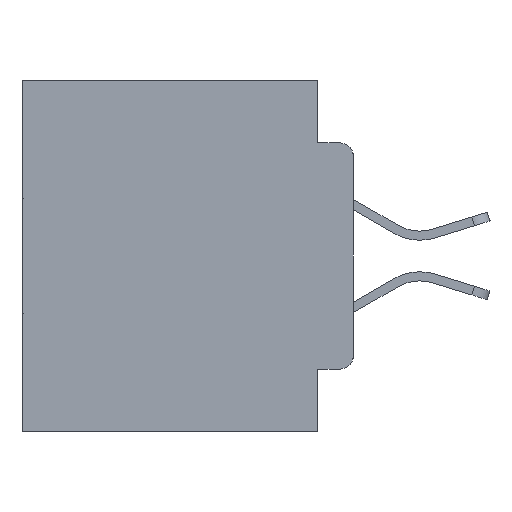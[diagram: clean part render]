
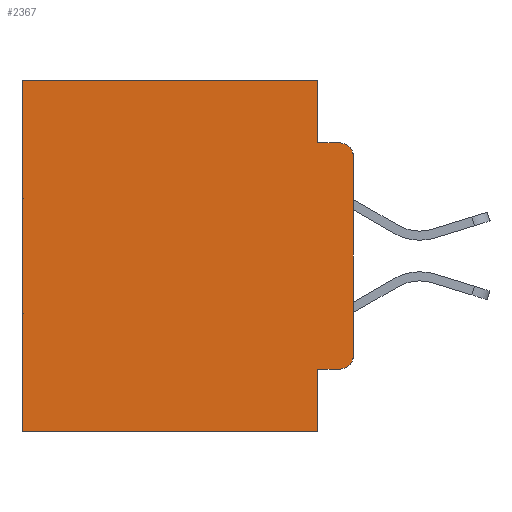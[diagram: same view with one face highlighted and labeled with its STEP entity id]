
A CAD part, left-side view. The second image highlights one B-rep face of the part: STEP entity #2367.
In plain terms, the highlighted planar face has unit normal (-1, 0, 0).
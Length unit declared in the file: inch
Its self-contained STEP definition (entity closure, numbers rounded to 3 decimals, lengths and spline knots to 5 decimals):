
#1033 = VECTOR ( 'NONE', #5697, 39.37008 ) ;
#1277 = EDGE_CURVE ( 'NONE', #19960, #2968, #4929, .T. ) ;
#1379 = CARTESIAN_POINT ( 'NONE',  ( 0.298, 0.051, 0. ) ) ;
#1910 = LINE ( 'NONE', #29981, #6306 ) ;
#2284 = ORIENTED_EDGE ( 'NONE', *, *, #23521, .T. ) ;
#2367 = ADVANCED_FACE ( 'NONE', ( #18465 ), #13854, .F. ) ;
#2561 = EDGE_CURVE ( 'NONE', #17976, #5956, #28846, .T. ) ;
#2610 = DIRECTION ( 'NONE',  ( -1., 0., 0. ) ) ;
#2968 = VERTEX_POINT ( 'NONE', #10141 ) ;
#3002 = AXIS2_PLACEMENT_3D ( 'NONE', #29935, #8965, #18314 ) ;
#3063 = VERTEX_POINT ( 'NONE', #20536 ) ;
#4716 = DIRECTION ( 'NONE',  ( -1., 0., 0. ) ) ;
#4929 = CIRCLE ( 'NONE', #16706, 0.02 ) ;
#5697 = DIRECTION ( 'NONE',  ( 0., 0., -1. ) ) ;
#5956 = VERTEX_POINT ( 'NONE', #21633 ) ;
#6157 = LINE ( 'NONE', #19961, #22907 ) ;
#6292 = EDGE_LOOP ( 'NONE', ( #26105, #29498, #7298, #27615, #23165, #8269, #11264, #27363, #2284, #11113 ) ) ;
#6306 = VECTOR ( 'NONE', #11306, 39.37008 ) ;
#6363 = CARTESIAN_POINT ( 'NONE',  ( 0.298, 0.051, -0.0885 ) ) ;
#6439 = CARTESIAN_POINT ( 'NONE',  ( 0.298, 0.051, 0. ) ) ;
#7035 = DIRECTION ( 'NONE',  ( 0., 0., -1. ) ) ;
#7298 = ORIENTED_EDGE ( 'NONE', *, *, #22353, .F. ) ;
#7480 = VERTEX_POINT ( 'NONE', #16252 ) ;
#8063 = VECTOR ( 'NONE', #23397, 39.37008 ) ;
#8269 = ORIENTED_EDGE ( 'NONE', *, *, #20281, .T. ) ;
#8716 = CARTESIAN_POINT ( 'NONE',  ( 0.298, 0., 0. ) ) ;
#8837 = CARTESIAN_POINT ( 'NONE',  ( 0.298, 0.473, 0. ) ) ;
#8862 = LINE ( 'NONE', #8716, #11197 ) ;
#8965 = DIRECTION ( 'NONE',  ( 1., 0., 0. ) ) ;
#9868 = CIRCLE ( 'NONE', #13774, 0.02 ) ;
#10141 = CARTESIAN_POINT ( 'NONE',  ( 0.298, 0.02, -0.0885 ) ) ;
#10756 = CARTESIAN_POINT ( 'NONE',  ( 0.298, 0., -0.3915 ) ) ;
#11113 = ORIENTED_EDGE ( 'NONE', *, *, #27445, .T. ) ;
#11197 = VECTOR ( 'NONE', #11311, 39.37008 ) ;
#11264 = ORIENTED_EDGE ( 'NONE', *, *, #23766, .F. ) ;
#11306 = DIRECTION ( 'NONE',  ( 0., 0., -1. ) ) ;
#11311 = DIRECTION ( 'NONE',  ( 0., 0., -1. ) ) ;
#11422 = EDGE_CURVE ( 'NONE', #17976, #7480, #6157, .T. ) ;
#11603 = CARTESIAN_POINT ( 'NONE',  ( 0.298, 0., -0.5 ) ) ;
#12415 = VERTEX_POINT ( 'NONE', #21894 ) ;
#12444 = EDGE_CURVE ( 'NONE', #18455, #3063, #1910, .T. ) ;
#13774 = AXIS2_PLACEMENT_3D ( 'NONE', #27733, #4716, #7035 ) ;
#13854 = PLANE ( 'NONE',  #3002 ) ;
#13896 = EDGE_CURVE ( 'NONE', #19960, #15166, #8862, .T. ) ;
#14668 = LINE ( 'NONE', #6363, #25718 ) ;
#15166 = VERTEX_POINT ( 'NONE', #10756 ) ;
#16252 = CARTESIAN_POINT ( 'NONE',  ( 0.298, 0.473, 0. ) ) ;
#16455 = VERTEX_POINT ( 'NONE', #28830 ) ;
#16706 = AXIS2_PLACEMENT_3D ( 'NONE', #23657, #2610, #28388 ) ;
#17124 = DIRECTION ( 'NONE',  ( 0., -1., 0. ) ) ;
#17976 = VERTEX_POINT ( 'NONE', #6439 ) ;
#18183 = DIRECTION ( 'NONE',  ( 0., 0., -1. ) ) ;
#18314 = DIRECTION ( 'NONE',  ( 0., 0., -1. ) ) ;
#18455 = VERTEX_POINT ( 'NONE', #20823 ) ;
#18465 = FACE_OUTER_BOUND ( 'NONE', #6292, .T. ) ;
#19960 = VERTEX_POINT ( 'NONE', #24024 ) ;
#19961 = CARTESIAN_POINT ( 'NONE',  ( 0.298, 0., 0. ) ) ;
#20281 = EDGE_CURVE ( 'NONE', #7480, #12415, #29815, .T. ) ;
#20536 = CARTESIAN_POINT ( 'NONE',  ( 0.298, 0.051, -0.5 ) ) ;
#20565 = DIRECTION ( 'NONE',  ( 0., 1., 0. ) ) ;
#20823 = CARTESIAN_POINT ( 'NONE',  ( 0.298, 0.051, -0.4115 ) ) ;
#21633 = CARTESIAN_POINT ( 'NONE',  ( 0.298, 0.051, -0.0885 ) ) ;
#21894 = CARTESIAN_POINT ( 'NONE',  ( 0.298, 0.473, -0.5 ) ) ;
#22257 = VECTOR ( 'NONE', #17124, 39.37008 ) ;
#22353 = EDGE_CURVE ( 'NONE', #5956, #2968, #14668, .T. ) ;
#22907 = VECTOR ( 'NONE', #20565, 39.37008 ) ;
#23165 = ORIENTED_EDGE ( 'NONE', *, *, #11422, .T. ) ;
#23397 = DIRECTION ( 'NONE',  ( 0., 1., 0. ) ) ;
#23521 = EDGE_CURVE ( 'NONE', #18455, #16455, #29219, .T. ) ;
#23657 = CARTESIAN_POINT ( 'NONE',  ( 0.298, 0.02, -0.1085 ) ) ;
#23766 = EDGE_CURVE ( 'NONE', #3063, #12415, #29964, .T. ) ;
#24024 = CARTESIAN_POINT ( 'NONE',  ( 0.298, 0., -0.1085 ) ) ;
#25718 = VECTOR ( 'NONE', #29806, 39.37008 ) ;
#26105 = ORIENTED_EDGE ( 'NONE', *, *, #13896, .F. ) ;
#26620 = CARTESIAN_POINT ( 'NONE',  ( 0.298, 0.051, -0.4115 ) ) ;
#27363 = ORIENTED_EDGE ( 'NONE', *, *, #12444, .F. ) ;
#27445 = EDGE_CURVE ( 'NONE', #16455, #15166, #9868, .T. ) ;
#27615 = ORIENTED_EDGE ( 'NONE', *, *, #2561, .F. ) ;
#27733 = CARTESIAN_POINT ( 'NONE',  ( 0.298, 0.02, -0.3915 ) ) ;
#28388 = DIRECTION ( 'NONE',  ( 0., 0., -1. ) ) ;
#28830 = CARTESIAN_POINT ( 'NONE',  ( 0.298, 0.02, -0.4115 ) ) ;
#28846 = LINE ( 'NONE', #1379, #1033 ) ;
#29219 = LINE ( 'NONE', #26620, #22257 ) ;
#29498 = ORIENTED_EDGE ( 'NONE', *, *, #1277, .T. ) ;
#29806 = DIRECTION ( 'NONE',  ( 0., -1., 0. ) ) ;
#29815 = LINE ( 'NONE', #8837, #29977 ) ;
#29935 = CARTESIAN_POINT ( 'NONE',  ( 0.298, 0., 0. ) ) ;
#29964 = LINE ( 'NONE', #11603, #8063 ) ;
#29977 = VECTOR ( 'NONE', #18183, 39.37008 ) ;
#29981 = CARTESIAN_POINT ( 'NONE',  ( 0.298, 0.051, 0. ) ) ;
